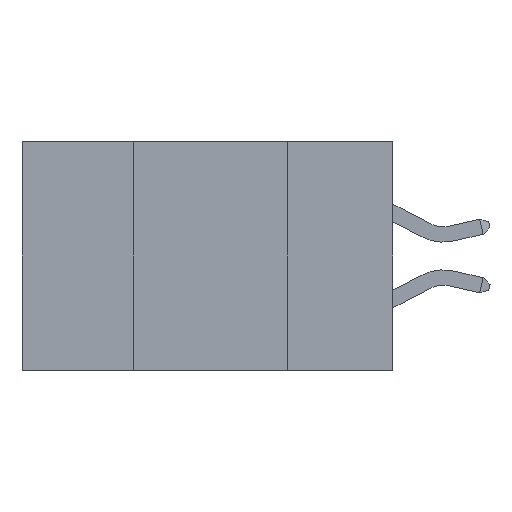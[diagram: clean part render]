
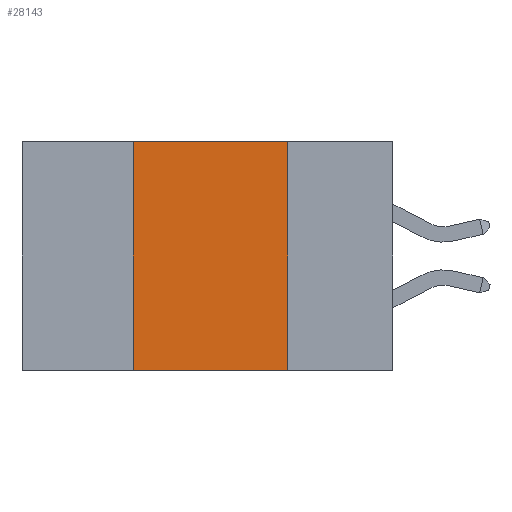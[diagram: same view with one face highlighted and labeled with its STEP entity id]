
A CAD part, left-side view. The second image highlights one B-rep face of the part: STEP entity #28143.
In plain terms, the highlighted planar face has unit normal (-1, 0, 0).
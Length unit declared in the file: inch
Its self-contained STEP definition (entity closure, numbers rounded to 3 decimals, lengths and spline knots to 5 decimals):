
#1725 = VERTEX_POINT ( 'NONE', #9903 ) ;
#2624 = VECTOR ( 'NONE', #9449, 39.37008 ) ;
#3553 = ORIENTED_EDGE ( 'NONE', *, *, #34403, .T. ) ;
#4460 = LINE ( 'NONE', #16175, #44033 ) ;
#5983 = DIRECTION ( 'NONE',  ( 0., -1., 0. ) ) ;
#6231 = CARTESIAN_POINT ( 'NONE',  ( 0., 0.17, 0. ) ) ;
#8584 = PLANE ( 'NONE',  #24707 ) ;
#9128 = VECTOR ( 'NONE', #23948, 39.37008 ) ;
#9449 = DIRECTION ( 'NONE',  ( 0., -1., 0. ) ) ;
#9903 = CARTESIAN_POINT ( 'NONE',  ( 0., 0.17, -0.37 ) ) ;
#13888 = CARTESIAN_POINT ( 'NONE',  ( 0., 0.42, 0. ) ) ;
#13945 = ORIENTED_EDGE ( 'NONE', *, *, #18636, .F. ) ;
#15333 = CARTESIAN_POINT ( 'NONE',  ( 0., 0.6, 0. ) ) ;
#15618 = DIRECTION ( 'NONE',  ( 0., 0., -1. ) ) ;
#16175 = CARTESIAN_POINT ( 'NONE',  ( 0., 0.6, -0.37 ) ) ;
#17503 = EDGE_CURVE ( 'NONE', #19349, #1725, #32138, .T. ) ;
#18092 = ORIENTED_EDGE ( 'NONE', *, *, #17503, .F. ) ;
#18629 = DIRECTION ( 'NONE',  ( 1., 0., 0. ) ) ;
#18636 = EDGE_CURVE ( 'NONE', #36430, #19349, #36839, .T. ) ;
#18822 = EDGE_CURVE ( 'NONE', #34471, #36430, #21868, .T. ) ;
#19175 = VECTOR ( 'NONE', #34246, 39.37008 ) ;
#19349 = VERTEX_POINT ( 'NONE', #6231 ) ;
#21868 = LINE ( 'NONE', #13888, #19175 ) ;
#23948 = DIRECTION ( 'NONE',  ( 0., 0., -1. ) ) ;
#24707 = AXIS2_PLACEMENT_3D ( 'NONE', #15333, #18629, #15618 ) ;
#28143 = ADVANCED_FACE ( 'NONE', ( #40649 ), #8584, .F. ) ;
#28813 = CARTESIAN_POINT ( 'NONE',  ( 0., 0.42, 0. ) ) ;
#30480 = CARTESIAN_POINT ( 'NONE',  ( 0., 0.17, 0. ) ) ;
#32138 = LINE ( 'NONE', #30480, #9128 ) ;
#32850 = EDGE_LOOP ( 'NONE', ( #18092, #13945, #36687, #3553 ) ) ;
#34246 = DIRECTION ( 'NONE',  ( 0., 0., 1. ) ) ;
#34403 = EDGE_CURVE ( 'NONE', #34471, #1725, #4460, .T. ) ;
#34471 = VERTEX_POINT ( 'NONE', #40200 ) ;
#36430 = VERTEX_POINT ( 'NONE', #28813 ) ;
#36687 = ORIENTED_EDGE ( 'NONE', *, *, #18822, .F. ) ;
#36839 = LINE ( 'NONE', #40647, #2624 ) ;
#40200 = CARTESIAN_POINT ( 'NONE',  ( 0., 0.42, -0.37 ) ) ;
#40647 = CARTESIAN_POINT ( 'NONE',  ( 0., 0.6, 0. ) ) ;
#40649 = FACE_OUTER_BOUND ( 'NONE', #32850, .T. ) ;
#44033 = VECTOR ( 'NONE', #5983, 39.37008 ) ;
